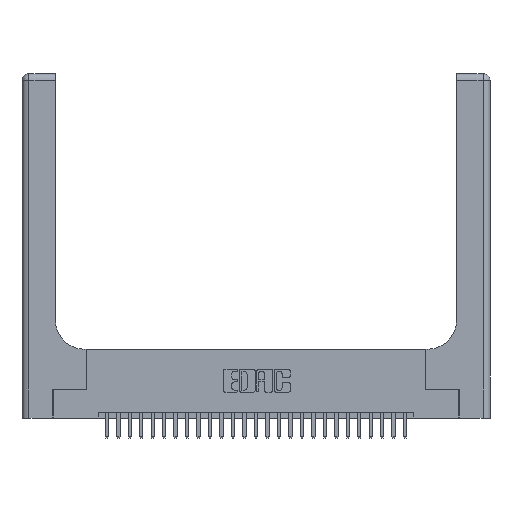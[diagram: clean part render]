
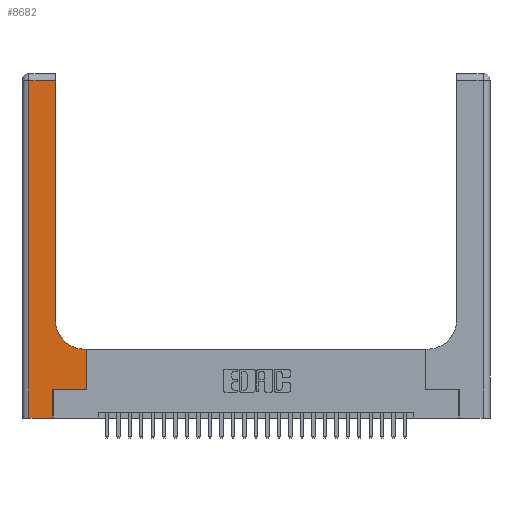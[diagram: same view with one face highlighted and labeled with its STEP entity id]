
A CAD part, top view. The second image highlights one B-rep face of the part: STEP entity #8682.
In plain terms, the highlighted planar face has unit normal (0, 0, 1).
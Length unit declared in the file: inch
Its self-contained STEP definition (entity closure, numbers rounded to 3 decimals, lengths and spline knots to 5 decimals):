
#1035 = VERTEX_POINT ( 'NONE', #10814 ) ;
#1113 = DIRECTION ( 'NONE',  ( -1., 0., 0. ) ) ;
#2157 = EDGE_CURVE ( 'NONE', #15101, #15064, #13179, .T. ) ;
#2539 = DIRECTION ( 'NONE',  ( 0., 1., 0. ) ) ;
#2875 = DIRECTION ( 'NONE',  ( 1., 0., 0. ) ) ;
#3405 = CARTESIAN_POINT ( 'NONE',  ( 0., 3., 0.37 ) ) ;
#3501 = DIRECTION ( 'NONE',  ( -1., 0., 0. ) ) ;
#4165 = CARTESIAN_POINT ( 'NONE',  ( 0.5415, 0.6, 0.37 ) ) ;
#4820 = LINE ( 'NONE', #20985, #23805 ) ;
#5134 = CARTESIAN_POINT ( 'NONE',  ( 0., 2.94, 0.37 ) ) ;
#5621 = CARTESIAN_POINT ( 'NONE',  ( 0.2915, 3., 0.37 ) ) ;
#5716 = ORIENTED_EDGE ( 'NONE', *, *, #21800, .T. ) ;
#5797 = DIRECTION ( 'NONE',  ( 0., 0., -1. ) ) ;
#6582 = LINE ( 'NONE', #5134, #7981 ) ;
#6630 = VERTEX_POINT ( 'NONE', #4165 ) ;
#6794 = CARTESIAN_POINT ( 'NONE',  ( 0.269, 0.25, 0.37 ) ) ;
#7218 = ORIENTED_EDGE ( 'NONE', *, *, #19718, .T. ) ;
#7495 = DIRECTION ( 'NONE',  ( 0., 0., -1. ) ) ;
#7981 = VECTOR ( 'NONE', #1113, 39.37008 ) ;
#8648 = ORIENTED_EDGE ( 'NONE', *, *, #19800, .T. ) ;
#8682 = ADVANCED_FACE ( 'NONE', ( #10558 ), #16563, .F. ) ;
#8837 = LINE ( 'NONE', #5621, #16452 ) ;
#9281 = EDGE_CURVE ( 'NONE', #6630, #21795, #27394, .T. ) ;
#9309 = ORIENTED_EDGE ( 'NONE', *, *, #2157, .T. ) ;
#9419 = EDGE_LOOP ( 'NONE', ( #23190, #18051, #19571, #9642, #5716, #9309, #7218, #8648, #20687 ) ) ;
#9499 = EDGE_CURVE ( 'NONE', #27233, #14104, #12579, .T. ) ;
#9642 = ORIENTED_EDGE ( 'NONE', *, *, #25228, .T. ) ;
#10558 = FACE_OUTER_BOUND ( 'NONE', #9419, .T. ) ;
#10814 = CARTESIAN_POINT ( 'NONE',  ( 0.5585, 0.6, 0.37 ) ) ;
#11168 = EDGE_CURVE ( 'NONE', #15440, #27233, #6582, .T. ) ;
#11463 = DIRECTION ( 'NONE',  ( 1., 0., 0. ) ) ;
#11711 = CARTESIAN_POINT ( 'NONE',  ( 0.5585, 0.25, 0.37 ) ) ;
#12510 = CARTESIAN_POINT ( 'NONE',  ( 0.269, 0.25, 0.37 ) ) ;
#12579 = LINE ( 'NONE', #18301, #16054 ) ;
#13179 = LINE ( 'NONE', #6794, #22139 ) ;
#13292 = CARTESIAN_POINT ( 'NONE',  ( 0.2915, 0.6, 0.37 ) ) ;
#13767 = CARTESIAN_POINT ( 'NONE',  ( 0.5415, 0.85, 0.37 ) ) ;
#14104 = VERTEX_POINT ( 'NONE', #15725 ) ;
#14899 = VERTEX_POINT ( 'NONE', #20968 ) ;
#14934 = VECTOR ( 'NONE', #21691, 39.37008 ) ;
#14993 = LINE ( 'NONE', #23102, #21537 ) ;
#15064 = VERTEX_POINT ( 'NONE', #16257 ) ;
#15101 = VERTEX_POINT ( 'NONE', #12510 ) ;
#15440 = VERTEX_POINT ( 'NONE', #27741 ) ;
#15725 = CARTESIAN_POINT ( 'NONE',  ( 0.06, 0., 0.37 ) ) ;
#15883 = DIRECTION ( 'NONE',  ( 0., -1., 0. ) ) ;
#16054 = VECTOR ( 'NONE', #15883, 39.37008 ) ;
#16257 = CARTESIAN_POINT ( 'NONE',  ( 0.5585, 0.25, 0.37 ) ) ;
#16452 = VECTOR ( 'NONE', #25758, 39.37008 ) ;
#16563 = PLANE ( 'NONE',  #23140 ) ;
#16679 = DIRECTION ( 'NONE',  ( 1., 0., 0. ) ) ;
#18051 = ORIENTED_EDGE ( 'NONE', *, *, #11168, .T. ) ;
#18151 = AXIS2_PLACEMENT_3D ( 'NONE', #13767, #7495, #2875 ) ;
#18301 = CARTESIAN_POINT ( 'NONE',  ( 0.06, 3., 0.37 ) ) ;
#19070 = VECTOR ( 'NONE', #2539, 39.37008 ) ;
#19558 = CARTESIAN_POINT ( 'NONE',  ( 0.06, 2.94, 0.37 ) ) ;
#19571 = ORIENTED_EDGE ( 'NONE', *, *, #9499, .T. ) ;
#19718 = EDGE_CURVE ( 'NONE', #15064, #1035, #23562, .T. ) ;
#19800 = EDGE_CURVE ( 'NONE', #1035, #6630, #24902, .T. ) ;
#20687 = ORIENTED_EDGE ( 'NONE', *, *, #9281, .T. ) ;
#20968 = CARTESIAN_POINT ( 'NONE',  ( 0.269, 0., 0.37 ) ) ;
#20985 = CARTESIAN_POINT ( 'NONE',  ( 0.269, 0., 0.37 ) ) ;
#21537 = VECTOR ( 'NONE', #16679, 39.37008 ) ;
#21691 = DIRECTION ( 'NONE',  ( -1., 0., 0. ) ) ;
#21795 = VERTEX_POINT ( 'NONE', #25593 ) ;
#21800 = EDGE_CURVE ( 'NONE', #14899, #15101, #4820, .T. ) ;
#22139 = VECTOR ( 'NONE', #11463, 39.37008 ) ;
#23102 = CARTESIAN_POINT ( 'NONE',  ( 0., 0., 0.37 ) ) ;
#23140 = AXIS2_PLACEMENT_3D ( 'NONE', #3405, #5797, #3501 ) ;
#23190 = ORIENTED_EDGE ( 'NONE', *, *, #27687, .T. ) ;
#23562 = LINE ( 'NONE', #11711, #19070 ) ;
#23805 = VECTOR ( 'NONE', #27507, 39.37008 ) ;
#24902 = LINE ( 'NONE', #13292, #14934 ) ;
#25228 = EDGE_CURVE ( 'NONE', #14104, #14899, #14993, .T. ) ;
#25593 = CARTESIAN_POINT ( 'NONE',  ( 0.2915, 0.85, 0.37 ) ) ;
#25758 = DIRECTION ( 'NONE',  ( 0., 1., 0. ) ) ;
#27233 = VERTEX_POINT ( 'NONE', #19558 ) ;
#27394 = CIRCLE ( 'NONE', #18151, 0.25 ) ;
#27507 = DIRECTION ( 'NONE',  ( 0., 1., 0. ) ) ;
#27687 = EDGE_CURVE ( 'NONE', #21795, #15440, #8837, .T. ) ;
#27741 = CARTESIAN_POINT ( 'NONE',  ( 0.2915, 2.94, 0.37 ) ) ;
